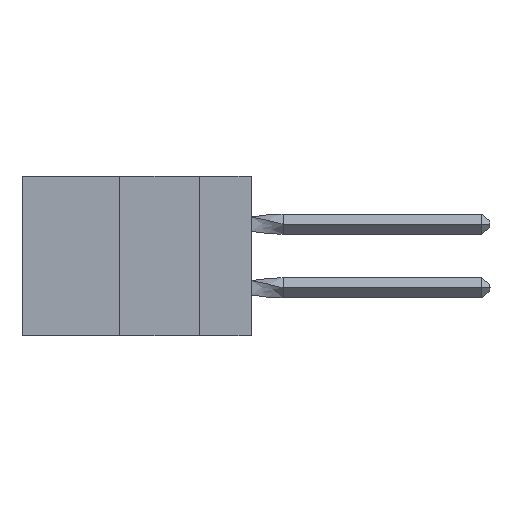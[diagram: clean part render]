
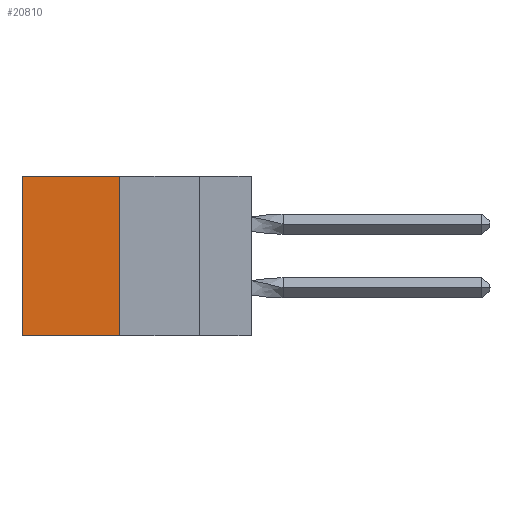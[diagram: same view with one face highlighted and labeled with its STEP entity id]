
A CAD part, left-side view. The second image highlights one B-rep face of the part: STEP entity #20810.
In plain terms, the highlighted planar face has unit normal (-1, 0, 0).
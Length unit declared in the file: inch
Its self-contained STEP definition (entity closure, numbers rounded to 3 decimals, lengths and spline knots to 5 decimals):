
#1574 = DIRECTION ( 'NONE',  ( 1., 0., 0. ) ) ;
#1738 = CARTESIAN_POINT ( 'NONE',  ( 0.305, 0.413, 0. ) ) ;
#2040 = EDGE_CURVE ( 'NONE', #9892, #15692, #19673, .T. ) ;
#2297 = CARTESIAN_POINT ( 'NONE',  ( 0.305, 0.72, 0. ) ) ;
#2331 = LINE ( 'NONE', #16436, #3941 ) ;
#3305 = DIRECTION ( 'NONE',  ( 0., 0., -1. ) ) ;
#3821 = DIRECTION ( 'NONE',  ( 0., 1., 0. ) ) ;
#3941 = VECTOR ( 'NONE', #3305, 39.37008 ) ;
#5433 = FACE_OUTER_BOUND ( 'NONE', #8960, .T. ) ;
#5722 = DIRECTION ( 'NONE',  ( 0., 0., -1. ) ) ;
#5730 = ORIENTED_EDGE ( 'NONE', *, *, #11261, .F. ) ;
#6593 = DIRECTION ( 'NONE',  ( 0., 1., 0. ) ) ;
#6648 = CARTESIAN_POINT ( 'NONE',  ( 0.305, 0.413, -0.5 ) ) ;
#6948 = EDGE_CURVE ( 'NONE', #14461, #18793, #2331, .T. ) ;
#8180 = CARTESIAN_POINT ( 'NONE',  ( 0.305, 0.413, -0.5 ) ) ;
#8244 = ORIENTED_EDGE ( 'NONE', *, *, #6948, .T. ) ;
#8960 = EDGE_LOOP ( 'NONE', ( #8244, #5730, #20475, #19999 ) ) ;
#9821 = VECTOR ( 'NONE', #3821, 39.37008 ) ;
#9850 = DIRECTION ( 'NONE',  ( 0., 0., -1. ) ) ;
#9892 = VERTEX_POINT ( 'NONE', #20143 ) ;
#10748 = CARTESIAN_POINT ( 'NONE',  ( 0.305, 0.72, -0.5 ) ) ;
#11261 = EDGE_CURVE ( 'NONE', #15692, #18793, #14412, .T. ) ;
#13895 = VECTOR ( 'NONE', #6593, 39.37008 ) ;
#14412 = LINE ( 'NONE', #8180, #13895 ) ;
#14461 = VERTEX_POINT ( 'NONE', #2297 ) ;
#14634 = PLANE ( 'NONE',  #18187 ) ;
#15240 = EDGE_CURVE ( 'NONE', #9892, #14461, #16030, .T. ) ;
#15692 = VERTEX_POINT ( 'NONE', #21247 ) ;
#16030 = LINE ( 'NONE', #1738, #9821 ) ;
#16436 = CARTESIAN_POINT ( 'NONE',  ( 0.305, 0.72, -0.5 ) ) ;
#18187 = AXIS2_PLACEMENT_3D ( 'NONE', #6648, #1574, #9850 ) ;
#18793 = VERTEX_POINT ( 'NONE', #10748 ) ;
#18902 = VECTOR ( 'NONE', #5722, 39.37008 ) ;
#19254 = CARTESIAN_POINT ( 'NONE',  ( 0.305, 0.413, -0.5 ) ) ;
#19673 = LINE ( 'NONE', #19254, #18902 ) ;
#19999 = ORIENTED_EDGE ( 'NONE', *, *, #15240, .T. ) ;
#20143 = CARTESIAN_POINT ( 'NONE',  ( 0.305, 0.413, 0. ) ) ;
#20475 = ORIENTED_EDGE ( 'NONE', *, *, #2040, .F. ) ;
#20810 = ADVANCED_FACE ( 'NONE', ( #5433 ), #14634, .F. ) ;
#21247 = CARTESIAN_POINT ( 'NONE',  ( 0.305, 0.413, -0.5 ) ) ;
